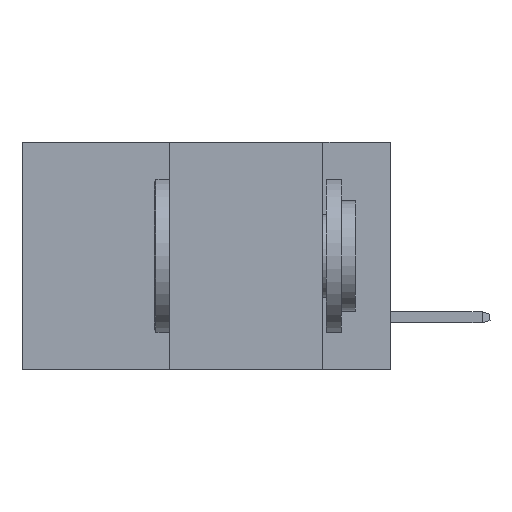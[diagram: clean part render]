
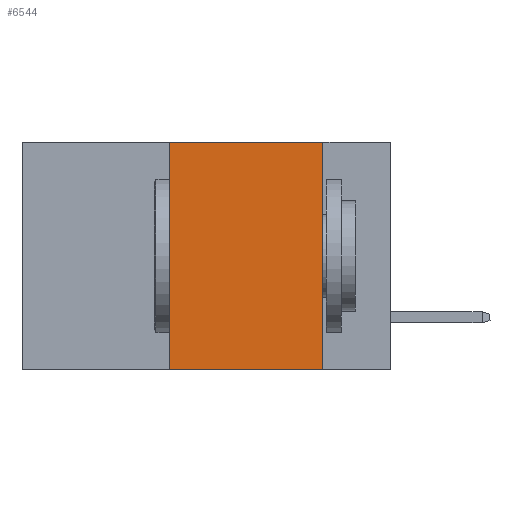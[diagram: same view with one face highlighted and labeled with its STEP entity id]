
A CAD part, left-side view. The second image highlights one B-rep face of the part: STEP entity #6544.
In plain terms, the highlighted planar face has unit normal (-1, 0, 0).
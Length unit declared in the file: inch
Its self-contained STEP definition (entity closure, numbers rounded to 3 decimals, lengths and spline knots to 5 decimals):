
#332 = EDGE_CURVE ( 'NONE', #12186, #5934, #8565, .T. ) ;
#1036 = LINE ( 'NONE', #11949, #1783 ) ;
#1582 = CARTESIAN_POINT ( 'NONE',  ( 0., 0.11, 0. ) ) ;
#1783 = VECTOR ( 'NONE', #5058, 39.37008 ) ;
#1909 = ORIENTED_EDGE ( 'NONE', *, *, #332, .F. ) ;
#2136 = LINE ( 'NONE', #1582, #14198 ) ;
#2333 = PLANE ( 'NONE',  #14018 ) ;
#2743 = LINE ( 'NONE', #9716, #12946 ) ;
#3045 = CARTESIAN_POINT ( 'NONE',  ( 0., 0.11, -0.37 ) ) ;
#3830 = VERTEX_POINT ( 'NONE', #13135 ) ;
#4233 = ORIENTED_EDGE ( 'NONE', *, *, #9682, .F. ) ;
#4836 = EDGE_CURVE ( 'NONE', #3830, #12186, #1036, .T. ) ;
#5058 = DIRECTION ( 'NONE',  ( 0., 0., 1. ) ) ;
#5382 = CARTESIAN_POINT ( 'NONE',  ( 0., 0.11, 0. ) ) ;
#5625 = VERTEX_POINT ( 'NONE', #3045 ) ;
#5934 = VERTEX_POINT ( 'NONE', #5382 ) ;
#6012 = VECTOR ( 'NONE', #7151, 39.37008 ) ;
#6074 = DIRECTION ( 'NONE',  ( 1., 0., 0. ) ) ;
#6544 = ADVANCED_FACE ( 'NONE', ( #9844 ), #2333, .F. ) ;
#7151 = DIRECTION ( 'NONE',  ( 0., -1., 0. ) ) ;
#7158 = CARTESIAN_POINT ( 'NONE',  ( 0., 0.36, 0. ) ) ;
#7474 = ORIENTED_EDGE ( 'NONE', *, *, #13814, .T. ) ;
#8552 = CARTESIAN_POINT ( 'NONE',  ( 0., 0.6, 0. ) ) ;
#8565 = LINE ( 'NONE', #8552, #6012 ) ;
#8811 = EDGE_LOOP ( 'NONE', ( #4233, #1909, #12265, #7474 ) ) ;
#9682 = EDGE_CURVE ( 'NONE', #5934, #5625, #2136, .T. ) ;
#9716 = CARTESIAN_POINT ( 'NONE',  ( 0., 0.6, -0.37 ) ) ;
#9844 = FACE_OUTER_BOUND ( 'NONE', #8811, .T. ) ;
#10570 = DIRECTION ( 'NONE',  ( 0., 0., -1. ) ) ;
#10850 = DIRECTION ( 'NONE',  ( 0., 0., -1. ) ) ;
#10857 = DIRECTION ( 'NONE',  ( 0., -1., 0. ) ) ;
#11949 = CARTESIAN_POINT ( 'NONE',  ( 0., 0.36, 0. ) ) ;
#12186 = VERTEX_POINT ( 'NONE', #7158 ) ;
#12265 = ORIENTED_EDGE ( 'NONE', *, *, #4836, .F. ) ;
#12946 = VECTOR ( 'NONE', #10857, 39.37008 ) ;
#13135 = CARTESIAN_POINT ( 'NONE',  ( 0., 0.36, -0.37 ) ) ;
#13814 = EDGE_CURVE ( 'NONE', #3830, #5625, #2743, .T. ) ;
#14018 = AXIS2_PLACEMENT_3D ( 'NONE', #15162, #6074, #10570 ) ;
#14198 = VECTOR ( 'NONE', #10850, 39.37008 ) ;
#15162 = CARTESIAN_POINT ( 'NONE',  ( 0., 0.6, 0. ) ) ;
